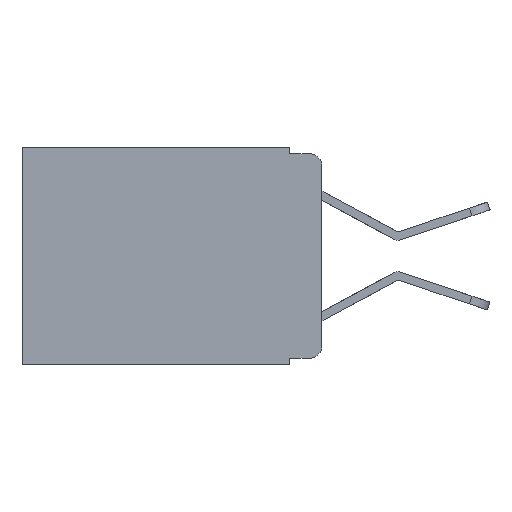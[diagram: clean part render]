
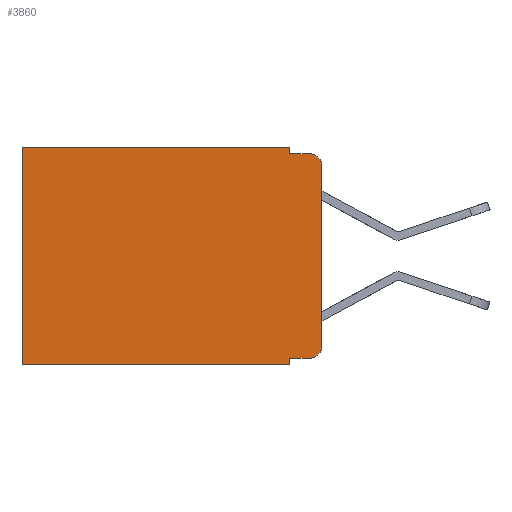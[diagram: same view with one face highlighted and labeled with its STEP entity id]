
A CAD part, left-side view. The second image highlights one B-rep face of the part: STEP entity #3860.
In plain terms, the highlighted planar face has unit normal (-1, 0, 0).
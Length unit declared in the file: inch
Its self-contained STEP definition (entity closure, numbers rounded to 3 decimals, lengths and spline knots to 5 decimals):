
#46 = EDGE_CURVE ( 'NONE', #12078, #13308, #10940, .T. ) ;
#155 = VECTOR ( 'NONE', #16086, 39.37008 ) ;
#338 = LINE ( 'NONE', #15989, #13636 ) ;
#339 = ORIENTED_EDGE ( 'NONE', *, *, #46, .F. ) ;
#604 = ORIENTED_EDGE ( 'NONE', *, *, #14185, .T. ) ;
#606 = LINE ( 'NONE', #8905, #7209 ) ;
#1071 = CARTESIAN_POINT ( 'NONE',  ( 0.298, 0.051, 0. ) ) ;
#1190 = CARTESIAN_POINT ( 'NONE',  ( 0.298, 0.051, -0.333 ) ) ;
#2059 = LINE ( 'NONE', #6327, #14762 ) ;
#2147 = VERTEX_POINT ( 'NONE', #1190 ) ;
#2180 = VERTEX_POINT ( 'NONE', #13373 ) ;
#2457 = LINE ( 'NONE', #14072, #12214 ) ;
#2483 = ORIENTED_EDGE ( 'NONE', *, *, #13356, .F. ) ;
#2686 = CARTESIAN_POINT ( 'NONE',  ( 0.298, 0.051, -0.01 ) ) ;
#2723 = DIRECTION ( 'NONE',  ( 0., 0., -1. ) ) ;
#2748 = VERTEX_POINT ( 'NONE', #9357 ) ;
#2774 = AXIS2_PLACEMENT_3D ( 'NONE', #6806, #15489, #8072 ) ;
#3102 = VERTEX_POINT ( 'NONE', #6438 ) ;
#3269 = CARTESIAN_POINT ( 'NONE',  ( 0.298, 0., 0. ) ) ;
#3385 = VERTEX_POINT ( 'NONE', #1071 ) ;
#3562 = CARTESIAN_POINT ( 'NONE',  ( 0.298, 0.02, -0.313 ) ) ;
#3842 = VECTOR ( 'NONE', #11331, 39.37008 ) ;
#3860 = ADVANCED_FACE ( 'NONE', ( #13765 ), #6028, .F. ) ;
#3878 = VERTEX_POINT ( 'NONE', #11822 ) ;
#4289 = CARTESIAN_POINT ( 'NONE',  ( 0.298, 0.051, -0.333 ) ) ;
#4545 = DIRECTION ( 'NONE',  ( 0., 0., -1. ) ) ;
#5079 = CARTESIAN_POINT ( 'NONE',  ( 0.298, 0.473, 0. ) ) ;
#5273 = CIRCLE ( 'NONE', #2774, 0.02 ) ;
#5777 = ORIENTED_EDGE ( 'NONE', *, *, #5826, .T. ) ;
#5826 = EDGE_CURVE ( 'NONE', #3878, #13308, #12154, .T. ) ;
#6028 = PLANE ( 'NONE',  #13629 ) ;
#6327 = CARTESIAN_POINT ( 'NONE',  ( 0.298, 0.473, 0. ) ) ;
#6343 = ORIENTED_EDGE ( 'NONE', *, *, #6632, .T. ) ;
#6412 = AXIS2_PLACEMENT_3D ( 'NONE', #3562, #12069, #4545 ) ;
#6438 = CARTESIAN_POINT ( 'NONE',  ( 0.298, 0.051, -0.01 ) ) ;
#6632 = EDGE_CURVE ( 'NONE', #2147, #3878, #15202, .T. ) ;
#6806 = CARTESIAN_POINT ( 'NONE',  ( 0.298, 0.02, -0.03 ) ) ;
#6856 = EDGE_CURVE ( 'NONE', #2180, #2748, #7230, .T. ) ;
#7116 = ORIENTED_EDGE ( 'NONE', *, *, #9154, .F. ) ;
#7209 = VECTOR ( 'NONE', #10150, 39.37008 ) ;
#7230 = LINE ( 'NONE', #13804, #3842 ) ;
#7332 = ORIENTED_EDGE ( 'NONE', *, *, #15311, .T. ) ;
#7401 = DIRECTION ( 'NONE',  ( 1., 0., 0. ) ) ;
#7432 = DIRECTION ( 'NONE',  ( 0., 0., -1. ) ) ;
#7946 = VERTEX_POINT ( 'NONE', #5079 ) ;
#8072 = DIRECTION ( 'NONE',  ( 0., 0., -1. ) ) ;
#8905 = CARTESIAN_POINT ( 'NONE',  ( 0.298, 0., 0. ) ) ;
#9019 = CARTESIAN_POINT ( 'NONE',  ( 0.298, 0., -0.03 ) ) ;
#9154 = EDGE_CURVE ( 'NONE', #2147, #2180, #338, .T. ) ;
#9357 = CARTESIAN_POINT ( 'NONE',  ( 0.298, 0.473, -0.343 ) ) ;
#9988 = EDGE_CURVE ( 'NONE', #7946, #2748, #2059, .T. ) ;
#10150 = DIRECTION ( 'NONE',  ( 0., 1., 0. ) ) ;
#10254 = ORIENTED_EDGE ( 'NONE', *, *, #9988, .T. ) ;
#10269 = DIRECTION ( 'NONE',  ( 0., -1., 0. ) ) ;
#10642 = VERTEX_POINT ( 'NONE', #11237 ) ;
#10756 = VECTOR ( 'NONE', #12923, 39.37008 ) ;
#10847 = EDGE_CURVE ( 'NONE', #3385, #3102, #2457, .T. ) ;
#10940 = LINE ( 'NONE', #12293, #155 ) ;
#11237 = CARTESIAN_POINT ( 'NONE',  ( 0.298, 0.02, -0.01 ) ) ;
#11331 = DIRECTION ( 'NONE',  ( 0., 1., 0. ) ) ;
#11822 = CARTESIAN_POINT ( 'NONE',  ( 0.298, 0.02, -0.333 ) ) ;
#12069 = DIRECTION ( 'NONE',  ( -1., 0., 0. ) ) ;
#12078 = VERTEX_POINT ( 'NONE', #9019 ) ;
#12154 = CIRCLE ( 'NONE', #6412, 0.02 ) ;
#12214 = VECTOR ( 'NONE', #2723, 39.37008 ) ;
#12293 = CARTESIAN_POINT ( 'NONE',  ( 0.298, 0., 0. ) ) ;
#12364 = DIRECTION ( 'NONE',  ( 0., 0., -1. ) ) ;
#12563 = DIRECTION ( 'NONE',  ( 0., 0., -1. ) ) ;
#12923 = DIRECTION ( 'NONE',  ( 0., -1., 0. ) ) ;
#13308 = VERTEX_POINT ( 'NONE', #16392 ) ;
#13356 = EDGE_CURVE ( 'NONE', #3102, #10642, #14099, .T. ) ;
#13373 = CARTESIAN_POINT ( 'NONE',  ( 0.298, 0.051, -0.343 ) ) ;
#13629 = AXIS2_PLACEMENT_3D ( 'NONE', #3269, #7401, #7432 ) ;
#13636 = VECTOR ( 'NONE', #12364, 39.37008 ) ;
#13719 = VECTOR ( 'NONE', #10269, 39.37008 ) ;
#13765 = FACE_OUTER_BOUND ( 'NONE', #16289, .T. ) ;
#13804 = CARTESIAN_POINT ( 'NONE',  ( 0.298, 0., -0.343 ) ) ;
#14072 = CARTESIAN_POINT ( 'NONE',  ( 0.298, 0.051, 0. ) ) ;
#14099 = LINE ( 'NONE', #2686, #13719 ) ;
#14185 = EDGE_CURVE ( 'NONE', #12078, #10642, #5273, .T. ) ;
#14762 = VECTOR ( 'NONE', #12563, 39.37008 ) ;
#14936 = ORIENTED_EDGE ( 'NONE', *, *, #6856, .F. ) ;
#15113 = ORIENTED_EDGE ( 'NONE', *, *, #10847, .F. ) ;
#15202 = LINE ( 'NONE', #4289, #10756 ) ;
#15311 = EDGE_CURVE ( 'NONE', #3385, #7946, #606, .T. ) ;
#15489 = DIRECTION ( 'NONE',  ( -1., 0., 0. ) ) ;
#15989 = CARTESIAN_POINT ( 'NONE',  ( 0.298, 0.051, 0. ) ) ;
#16086 = DIRECTION ( 'NONE',  ( 0., 0., -1. ) ) ;
#16289 = EDGE_LOOP ( 'NONE', ( #339, #604, #2483, #15113, #7332, #10254, #14936, #7116, #6343, #5777 ) ) ;
#16392 = CARTESIAN_POINT ( 'NONE',  ( 0.298, 0., -0.313 ) ) ;
